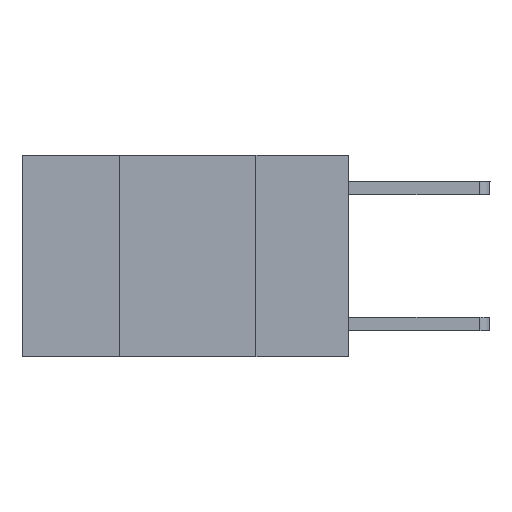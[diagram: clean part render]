
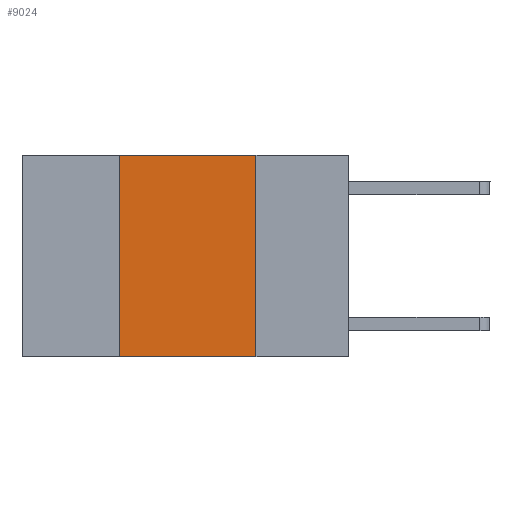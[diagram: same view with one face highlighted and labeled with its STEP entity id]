
A CAD part, left-side view. The second image highlights one B-rep face of the part: STEP entity #9024.
In plain terms, the highlighted planar face has unit normal (-1, 0, 0).
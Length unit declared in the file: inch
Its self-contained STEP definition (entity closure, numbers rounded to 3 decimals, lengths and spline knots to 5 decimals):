
#68 = VECTOR ( 'NONE', #4300, 39.37008 ) ;
#77 = LINE ( 'NONE', #7548, #369 ) ;
#369 = VECTOR ( 'NONE', #8280, 39.37008 ) ;
#1306 = DIRECTION ( 'NONE',  ( 0., 0., -1. ) ) ;
#1504 = VECTOR ( 'NONE', #4076, 39.37008 ) ;
#1576 = CARTESIAN_POINT ( 'NONE',  ( 0., 0.17, 0. ) ) ;
#1729 = VERTEX_POINT ( 'NONE', #3917 ) ;
#2252 = CARTESIAN_POINT ( 'NONE',  ( 0., 0.42, -0.37 ) ) ;
#2874 = CARTESIAN_POINT ( 'NONE',  ( 0., 0.42, 0. ) ) ;
#3068 = ORIENTED_EDGE ( 'NONE', *, *, #8109, .F. ) ;
#3469 = VERTEX_POINT ( 'NONE', #2874 ) ;
#3777 = EDGE_CURVE ( 'NONE', #9110, #3469, #10257, .T. ) ;
#3863 = DIRECTION ( 'NONE',  ( 0., -1., 0. ) ) ;
#3917 = CARTESIAN_POINT ( 'NONE',  ( 0., 0.17, 0. ) ) ;
#4076 = DIRECTION ( 'NONE',  ( 0., 0., -1. ) ) ;
#4300 = DIRECTION ( 'NONE',  ( 0., 0., 1. ) ) ;
#4514 = FACE_OUTER_BOUND ( 'NONE', #9265, .T. ) ;
#5362 = CARTESIAN_POINT ( 'NONE',  ( 0., 0.6, 0. ) ) ;
#5834 = LINE ( 'NONE', #1576, #1504 ) ;
#5958 = ORIENTED_EDGE ( 'NONE', *, *, #6901, .F. ) ;
#6000 = ORIENTED_EDGE ( 'NONE', *, *, #3777, .F. ) ;
#6101 = VECTOR ( 'NONE', #3863, 39.37008 ) ;
#6135 = ORIENTED_EDGE ( 'NONE', *, *, #7218, .T. ) ;
#6201 = PLANE ( 'NONE',  #9124 ) ;
#6237 = CARTESIAN_POINT ( 'NONE',  ( 0., 0.17, -0.37 ) ) ;
#6901 = EDGE_CURVE ( 'NONE', #1729, #9032, #5834, .T. ) ;
#7003 = DIRECTION ( 'NONE',  ( 1., 0., 0. ) ) ;
#7218 = EDGE_CURVE ( 'NONE', #9110, #9032, #10392, .T. ) ;
#7548 = CARTESIAN_POINT ( 'NONE',  ( 0., 0.6, 0. ) ) ;
#8109 = EDGE_CURVE ( 'NONE', #3469, #1729, #77, .T. ) ;
#8280 = DIRECTION ( 'NONE',  ( 0., -1., 0. ) ) ;
#9024 = ADVANCED_FACE ( 'NONE', ( #4514 ), #6201, .F. ) ;
#9032 = VERTEX_POINT ( 'NONE', #6237 ) ;
#9110 = VERTEX_POINT ( 'NONE', #2252 ) ;
#9124 = AXIS2_PLACEMENT_3D ( 'NONE', #5362, #7003, #1306 ) ;
#9265 = EDGE_LOOP ( 'NONE', ( #5958, #3068, #6000, #6135 ) ) ;
#9757 = CARTESIAN_POINT ( 'NONE',  ( 0., 0.42, 0. ) ) ;
#10133 = CARTESIAN_POINT ( 'NONE',  ( 0., 0.6, -0.37 ) ) ;
#10257 = LINE ( 'NONE', #9757, #68 ) ;
#10392 = LINE ( 'NONE', #10133, #6101 ) ;
